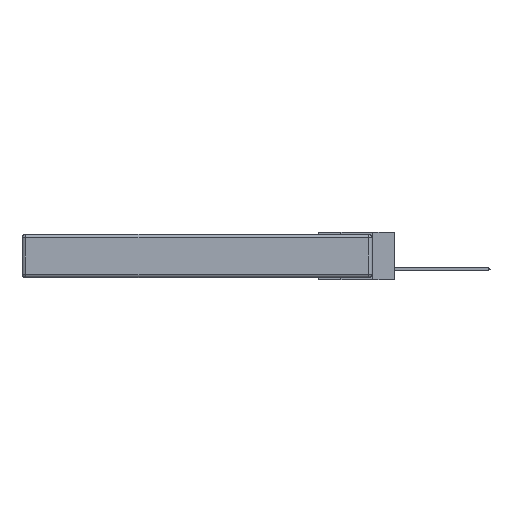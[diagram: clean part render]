
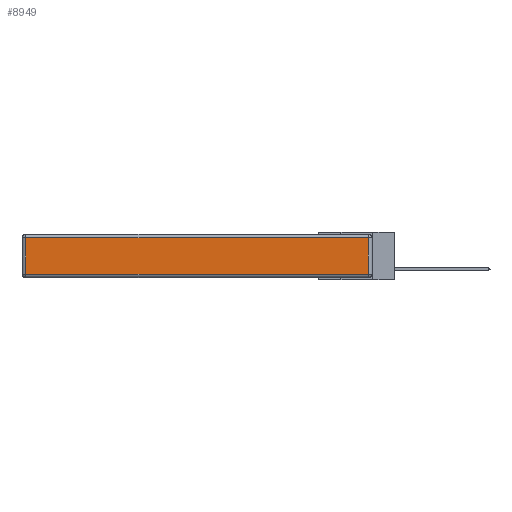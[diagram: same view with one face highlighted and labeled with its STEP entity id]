
A CAD part, left-side view. The second image highlights one B-rep face of the part: STEP entity #8949.
In plain terms, the highlighted planar face has unit normal (-1, 0, 0).
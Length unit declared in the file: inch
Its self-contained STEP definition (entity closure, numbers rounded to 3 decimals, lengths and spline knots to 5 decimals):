
#1090 = ORIENTED_EDGE ( 'NONE', *, *, #18411, .T. ) ;
#1370 = DIRECTION ( 'NONE',  ( 0., 1., 0. ) ) ;
#1932 = VECTOR ( 'NONE', #12779, 39.37008 ) ;
#2008 = DIRECTION ( 'NONE',  ( 0., -1., 0. ) ) ;
#2683 = VERTEX_POINT ( 'NONE', #17024 ) ;
#2882 = CARTESIAN_POINT ( 'NONE',  ( 0., 2.72, -0.313 ) ) ;
#2927 = CARTESIAN_POINT ( 'NONE',  ( 0., 0., -0.343 ) ) ;
#3208 = EDGE_CURVE ( 'NONE', #2683, #13928, #16213, .T. ) ;
#4079 = DIRECTION ( 'NONE',  ( 0., 0., -1. ) ) ;
#5863 = ORIENTED_EDGE ( 'NONE', *, *, #6096, .T. ) ;
#6096 = EDGE_CURVE ( 'NONE', #13928, #20511, #7687, .T. ) ;
#6489 = EDGE_LOOP ( 'NONE', ( #5863, #1090, #6744, #18032 ) ) ;
#6665 = CARTESIAN_POINT ( 'NONE',  ( 0., 0.03, -0.03 ) ) ;
#6744 = ORIENTED_EDGE ( 'NONE', *, *, #20701, .T. ) ;
#7555 = FACE_OUTER_BOUND ( 'NONE', #6489, .T. ) ;
#7652 = DIRECTION ( 'NONE',  ( -1., 0., 0. ) ) ;
#7687 = LINE ( 'NONE', #19855, #9432 ) ;
#7881 = CARTESIAN_POINT ( 'NONE',  ( 0., 0.03, -0.343 ) ) ;
#8949 = ADVANCED_FACE ( 'NONE', ( #7555 ), #12705, .T. ) ;
#9432 = VECTOR ( 'NONE', #2008, 39.37008 ) ;
#11888 = VECTOR ( 'NONE', #4079, 39.37008 ) ;
#12037 = VECTOR ( 'NONE', #1370, 39.37008 ) ;
#12569 = DIRECTION ( 'NONE',  ( 0., 0., 1. ) ) ;
#12705 = PLANE ( 'NONE',  #19084 ) ;
#12779 = DIRECTION ( 'NONE',  ( 0., 0., 1. ) ) ;
#13928 = VERTEX_POINT ( 'NONE', #2882 ) ;
#14256 = CARTESIAN_POINT ( 'NONE',  ( 0., 2.75, -0.03 ) ) ;
#16213 = LINE ( 'NONE', #17009, #11888 ) ;
#16376 = LINE ( 'NONE', #14256, #12037 ) ;
#17009 = CARTESIAN_POINT ( 'NONE',  ( 0., 2.72, -0.343 ) ) ;
#17024 = CARTESIAN_POINT ( 'NONE',  ( 0., 2.72, -0.03 ) ) ;
#18032 = ORIENTED_EDGE ( 'NONE', *, *, #3208, .T. ) ;
#18411 = EDGE_CURVE ( 'NONE', #20511, #19031, #18461, .T. ) ;
#18461 = LINE ( 'NONE', #7881, #1932 ) ;
#19031 = VERTEX_POINT ( 'NONE', #6665 ) ;
#19084 = AXIS2_PLACEMENT_3D ( 'NONE', #2927, #7652, #12569 ) ;
#19855 = CARTESIAN_POINT ( 'NONE',  ( 0., 0., -0.313 ) ) ;
#20295 = CARTESIAN_POINT ( 'NONE',  ( 0., 0.03, -0.313 ) ) ;
#20511 = VERTEX_POINT ( 'NONE', #20295 ) ;
#20701 = EDGE_CURVE ( 'NONE', #19031, #2683, #16376, .T. ) ;
